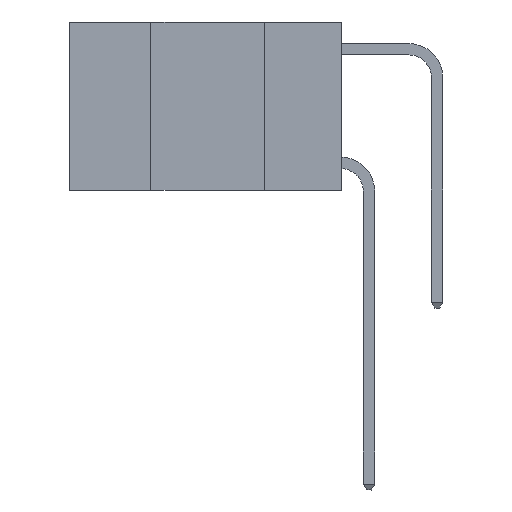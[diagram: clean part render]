
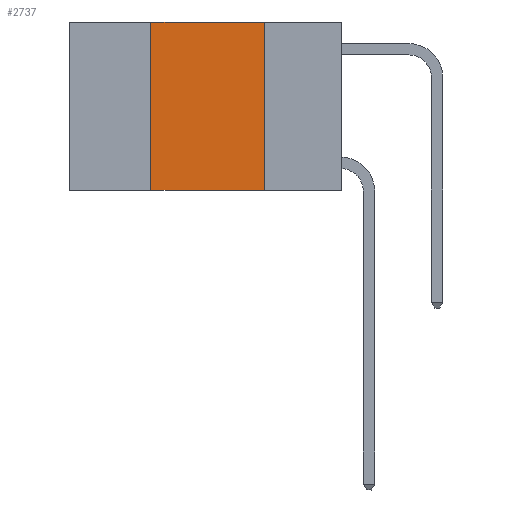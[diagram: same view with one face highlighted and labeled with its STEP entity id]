
A CAD part, left-side view. The second image highlights one B-rep face of the part: STEP entity #2737.
In plain terms, the highlighted planar face has unit normal (-1, 0, 0).
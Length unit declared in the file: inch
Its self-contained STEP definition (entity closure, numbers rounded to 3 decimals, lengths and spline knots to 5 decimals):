
#212 = EDGE_CURVE ( 'NONE', #5312, #1040, #4883, .T. ) ;
#735 = LINE ( 'NONE', #4764, #11780 ) ;
#1001 = ORIENTED_EDGE ( 'NONE', *, *, #1623, .T. ) ;
#1040 = VERTEX_POINT ( 'NONE', #5090 ) ;
#1623 = EDGE_CURVE ( 'NONE', #5312, #7797, #4871, .T. ) ;
#2478 = VECTOR ( 'NONE', #12022, 39.37008 ) ;
#2614 = PLANE ( 'NONE',  #3392 ) ;
#2737 = ADVANCED_FACE ( 'NONE', ( #4219 ), #2614, .F. ) ;
#2904 = EDGE_LOOP ( 'NONE', ( #4658, #4692, #4836, #1001 ) ) ;
#3392 = AXIS2_PLACEMENT_3D ( 'NONE', #7043, #3877, #9828 ) ;
#3765 = DIRECTION ( 'NONE',  ( 0., -1., 0. ) ) ;
#3877 = DIRECTION ( 'NONE',  ( 1., 0., 0. ) ) ;
#4219 = FACE_OUTER_BOUND ( 'NONE', #2904, .T. ) ;
#4547 = VERTEX_POINT ( 'NONE', #7823 ) ;
#4658 = ORIENTED_EDGE ( 'NONE', *, *, #9707, .F. ) ;
#4692 = ORIENTED_EDGE ( 'NONE', *, *, #7794, .F. ) ;
#4764 = CARTESIAN_POINT ( 'NONE',  ( 0., 0.17, 0. ) ) ;
#4836 = ORIENTED_EDGE ( 'NONE', *, *, #212, .F. ) ;
#4871 = LINE ( 'NONE', #12531, #6097 ) ;
#4883 = LINE ( 'NONE', #5131, #2478 ) ;
#5090 = CARTESIAN_POINT ( 'NONE',  ( 0., 0.42, 0. ) ) ;
#5131 = CARTESIAN_POINT ( 'NONE',  ( 0., 0.42, 0. ) ) ;
#5312 = VERTEX_POINT ( 'NONE', #10908 ) ;
#5869 = LINE ( 'NONE', #6774, #6840 ) ;
#6097 = VECTOR ( 'NONE', #3765, 39.37008 ) ;
#6635 = DIRECTION ( 'NONE',  ( 0., 0., -1. ) ) ;
#6774 = CARTESIAN_POINT ( 'NONE',  ( 0., 0.6, 0. ) ) ;
#6840 = VECTOR ( 'NONE', #10699, 39.37008 ) ;
#7043 = CARTESIAN_POINT ( 'NONE',  ( 0., 0.6, 0. ) ) ;
#7794 = EDGE_CURVE ( 'NONE', #1040, #4547, #5869, .T. ) ;
#7797 = VERTEX_POINT ( 'NONE', #11706 ) ;
#7823 = CARTESIAN_POINT ( 'NONE',  ( 0., 0.17, 0. ) ) ;
#9707 = EDGE_CURVE ( 'NONE', #4547, #7797, #735, .T. ) ;
#9828 = DIRECTION ( 'NONE',  ( 0., 0., -1. ) ) ;
#10699 = DIRECTION ( 'NONE',  ( 0., -1., 0. ) ) ;
#10908 = CARTESIAN_POINT ( 'NONE',  ( 0., 0.42, -0.37 ) ) ;
#11706 = CARTESIAN_POINT ( 'NONE',  ( 0., 0.17, -0.37 ) ) ;
#11780 = VECTOR ( 'NONE', #6635, 39.37008 ) ;
#12022 = DIRECTION ( 'NONE',  ( 0., 0., 1. ) ) ;
#12531 = CARTESIAN_POINT ( 'NONE',  ( 0., 0.6, -0.37 ) ) ;
